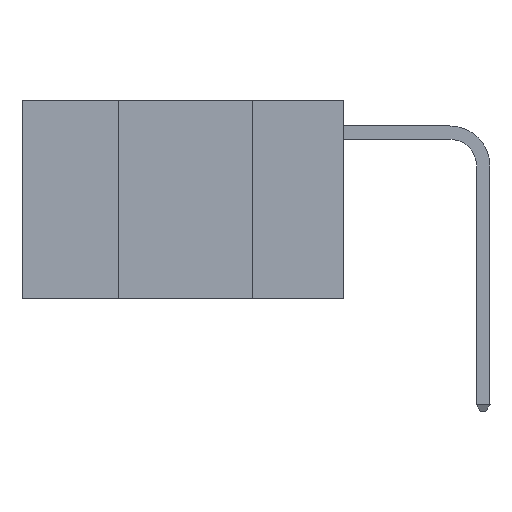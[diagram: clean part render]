
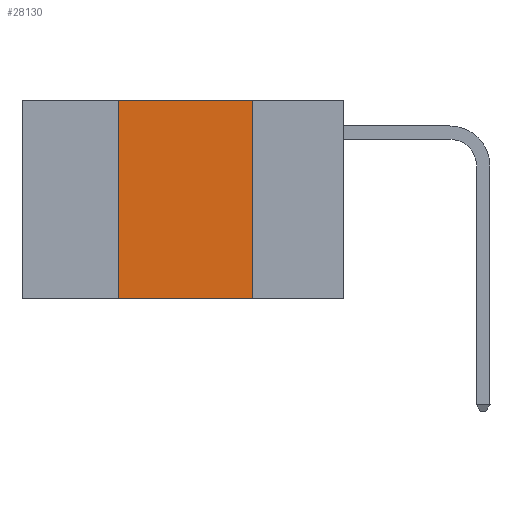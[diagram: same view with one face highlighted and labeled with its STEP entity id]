
A CAD part, left-side view. The second image highlights one B-rep face of the part: STEP entity #28130.
In plain terms, the highlighted planar face has unit normal (-1, 0, 0).
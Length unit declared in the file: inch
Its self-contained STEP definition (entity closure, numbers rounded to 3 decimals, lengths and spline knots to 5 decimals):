
#825 = LINE ( 'NONE', #3330, #10004 ) ;
#2072 = ORIENTED_EDGE ( 'NONE', *, *, #8127, .T. ) ;
#2298 = VERTEX_POINT ( 'NONE', #9290 ) ;
#2753 = DIRECTION ( 'NONE',  ( 0., -1., 0. ) ) ;
#3330 = CARTESIAN_POINT ( 'NONE',  ( 0., 0.6, -0.37 ) ) ;
#4110 = VERTEX_POINT ( 'NONE', #23173 ) ;
#4321 = CARTESIAN_POINT ( 'NONE',  ( 0., 0.17, 0. ) ) ;
#4665 = ORIENTED_EDGE ( 'NONE', *, *, #8844, .F. ) ;
#5934 = PLANE ( 'NONE',  #28975 ) ;
#6806 = LINE ( 'NONE', #4321, #8473 ) ;
#8127 = EDGE_CURVE ( 'NONE', #19239, #4110, #825, .T. ) ;
#8473 = VECTOR ( 'NONE', #28937, 39.37008 ) ;
#8630 = EDGE_CURVE ( 'NONE', #19239, #17891, #14081, .T. ) ;
#8791 = ORIENTED_EDGE ( 'NONE', *, *, #8841, .F. ) ;
#8841 = EDGE_CURVE ( 'NONE', #2298, #4110, #6806, .T. ) ;
#8844 = EDGE_CURVE ( 'NONE', #17891, #2298, #9037, .T. ) ;
#9037 = LINE ( 'NONE', #11111, #20711 ) ;
#9290 = CARTESIAN_POINT ( 'NONE',  ( 0., 0.17, 0. ) ) ;
#9363 = DIRECTION ( 'NONE',  ( 0., 0., 1. ) ) ;
#10004 = VECTOR ( 'NONE', #2753, 39.37008 ) ;
#11111 = CARTESIAN_POINT ( 'NONE',  ( 0., 0.6, 0. ) ) ;
#14081 = LINE ( 'NONE', #25434, #21404 ) ;
#17449 = CARTESIAN_POINT ( 'NONE',  ( 0., 0.6, 0. ) ) ;
#17459 = DIRECTION ( 'NONE',  ( 0., -1., 0. ) ) ;
#17587 = EDGE_LOOP ( 'NONE', ( #8791, #4665, #18803, #2072 ) ) ;
#17730 = DIRECTION ( 'NONE',  ( 0., 0., -1. ) ) ;
#17891 = VERTEX_POINT ( 'NONE', #18914 ) ;
#18803 = ORIENTED_EDGE ( 'NONE', *, *, #8630, .F. ) ;
#18914 = CARTESIAN_POINT ( 'NONE',  ( 0., 0.42, 0. ) ) ;
#18921 = CARTESIAN_POINT ( 'NONE',  ( 0., 0.42, -0.37 ) ) ;
#19239 = VERTEX_POINT ( 'NONE', #18921 ) ;
#20711 = VECTOR ( 'NONE', #17459, 39.37008 ) ;
#21404 = VECTOR ( 'NONE', #9363, 39.37008 ) ;
#23173 = CARTESIAN_POINT ( 'NONE',  ( 0., 0.17, -0.37 ) ) ;
#25434 = CARTESIAN_POINT ( 'NONE',  ( 0., 0.42, 0. ) ) ;
#26567 = DIRECTION ( 'NONE',  ( 1., 0., 0. ) ) ;
#28130 = ADVANCED_FACE ( 'NONE', ( #28346 ), #5934, .F. ) ;
#28346 = FACE_OUTER_BOUND ( 'NONE', #17587, .T. ) ;
#28937 = DIRECTION ( 'NONE',  ( 0., 0., -1. ) ) ;
#28975 = AXIS2_PLACEMENT_3D ( 'NONE', #17449, #26567, #17730 ) ;
